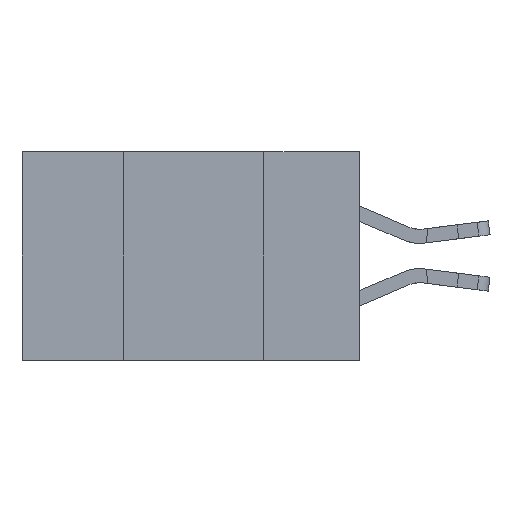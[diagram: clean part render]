
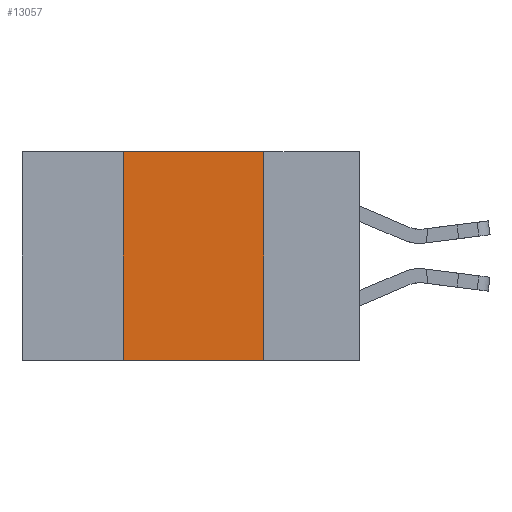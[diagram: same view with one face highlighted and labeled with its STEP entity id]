
A CAD part, left-side view. The second image highlights one B-rep face of the part: STEP entity #13057.
In plain terms, the highlighted planar face has unit normal (-1, 0, 0).
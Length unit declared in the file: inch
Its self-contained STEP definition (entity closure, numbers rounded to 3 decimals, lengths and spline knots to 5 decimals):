
#819 = CARTESIAN_POINT ( 'NONE',  ( 0., 0.17, -0.37 ) ) ;
#1199 = LINE ( 'NONE', #8742, #12016 ) ;
#1453 = LINE ( 'NONE', #11933, #3826 ) ;
#1654 = PLANE ( 'NONE',  #8919 ) ;
#3819 = EDGE_LOOP ( 'NONE', ( #11426, #14833, #16980, #23418 ) ) ;
#3826 = VECTOR ( 'NONE', #11844, 39.37008 ) ;
#5196 = VERTEX_POINT ( 'NONE', #14788 ) ;
#5303 = CARTESIAN_POINT ( 'NONE',  ( 0., 0.6, 0. ) ) ;
#6710 = DIRECTION ( 'NONE',  ( 0., -1., 0. ) ) ;
#8742 = CARTESIAN_POINT ( 'NONE',  ( 0., 0.42, 0. ) ) ;
#8919 = AXIS2_PLACEMENT_3D ( 'NONE', #13250, #23048, #19010 ) ;
#10814 = DIRECTION ( 'NONE',  ( 0., 0., -1. ) ) ;
#11426 = ORIENTED_EDGE ( 'NONE', *, *, #17022, .F. ) ;
#11455 = CARTESIAN_POINT ( 'NONE',  ( 0., 0.42, -0.37 ) ) ;
#11844 = DIRECTION ( 'NONE',  ( 0., -1., 0. ) ) ;
#11933 = CARTESIAN_POINT ( 'NONE',  ( 0., 0.6, -0.37 ) ) ;
#12016 = VECTOR ( 'NONE', #12735, 39.37008 ) ;
#12581 = FACE_OUTER_BOUND ( 'NONE', #3819, .T. ) ;
#12735 = DIRECTION ( 'NONE',  ( 0., 0., 1. ) ) ;
#13057 = ADVANCED_FACE ( 'NONE', ( #12581 ), #1654, .F. ) ;
#13250 = CARTESIAN_POINT ( 'NONE',  ( 0., 0.6, 0. ) ) ;
#14318 = VECTOR ( 'NONE', #10814, 39.37008 ) ;
#14788 = CARTESIAN_POINT ( 'NONE',  ( 0., 0.42, 0. ) ) ;
#14833 = ORIENTED_EDGE ( 'NONE', *, *, #22752, .F. ) ;
#14917 = LINE ( 'NONE', #16879, #14318 ) ;
#14976 = EDGE_CURVE ( 'NONE', #22317, #5196, #1199, .T. ) ;
#15143 = VECTOR ( 'NONE', #6710, 39.37008 ) ;
#16158 = VERTEX_POINT ( 'NONE', #819 ) ;
#16879 = CARTESIAN_POINT ( 'NONE',  ( 0., 0.17, 0. ) ) ;
#16980 = ORIENTED_EDGE ( 'NONE', *, *, #14976, .F. ) ;
#17022 = EDGE_CURVE ( 'NONE', #20510, #16158, #14917, .T. ) ;
#19010 = DIRECTION ( 'NONE',  ( 0., 0., -1. ) ) ;
#19830 = EDGE_CURVE ( 'NONE', #22317, #16158, #1453, .T. ) ;
#20211 = LINE ( 'NONE', #5303, #15143 ) ;
#20510 = VERTEX_POINT ( 'NONE', #23140 ) ;
#22317 = VERTEX_POINT ( 'NONE', #11455 ) ;
#22752 = EDGE_CURVE ( 'NONE', #5196, #20510, #20211, .T. ) ;
#23048 = DIRECTION ( 'NONE',  ( 1., 0., 0. ) ) ;
#23140 = CARTESIAN_POINT ( 'NONE',  ( 0., 0.17, 0. ) ) ;
#23418 = ORIENTED_EDGE ( 'NONE', *, *, #19830, .T. ) ;
